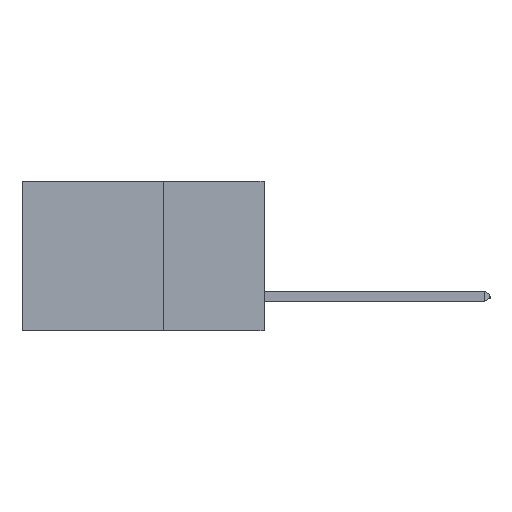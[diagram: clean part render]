
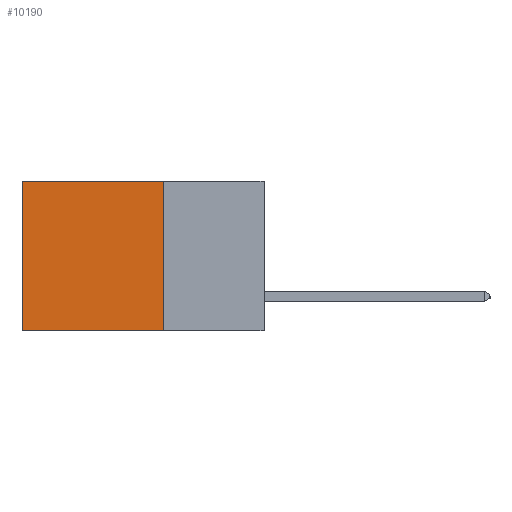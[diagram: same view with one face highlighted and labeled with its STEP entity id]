
A CAD part, left-side view. The second image highlights one B-rep face of the part: STEP entity #10190.
In plain terms, the highlighted planar face has unit normal (-1, 0, 0).
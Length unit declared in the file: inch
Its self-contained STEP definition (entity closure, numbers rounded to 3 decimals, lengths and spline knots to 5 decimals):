
#418 = DIRECTION ( 'NONE',  ( 0., 0., -1. ) ) ;
#2189 = LINE ( 'NONE', #14731, #21818 ) ;
#2745 = VECTOR ( 'NONE', #11582, 39.37008 ) ;
#2777 = VERTEX_POINT ( 'NONE', #9541 ) ;
#3739 = DIRECTION ( 'NONE',  ( 0., 1., 0. ) ) ;
#4799 = CARTESIAN_POINT ( 'NONE',  ( 0.298, 0.25, 0. ) ) ;
#5933 = EDGE_CURVE ( 'NONE', #11827, #14405, #5958, .T. ) ;
#5958 = LINE ( 'NONE', #19879, #7704 ) ;
#7068 = ORIENTED_EDGE ( 'NONE', *, *, #18054, .F. ) ;
#7145 = EDGE_CURVE ( 'NONE', #2777, #14405, #16252, .T. ) ;
#7150 = EDGE_LOOP ( 'NONE', ( #20111, #16093, #7068, #17313 ) ) ;
#7327 = CARTESIAN_POINT ( 'NONE',  ( 0.298, 0.25, 0. ) ) ;
#7704 = VECTOR ( 'NONE', #14851, 39.37008 ) ;
#9541 = CARTESIAN_POINT ( 'NONE',  ( 0.298, 0.25, -0.37 ) ) ;
#10190 = ADVANCED_FACE ( 'NONE', ( #22215 ), #18770, .F. ) ;
#11484 = DIRECTION ( 'NONE',  ( 1., 0., 0. ) ) ;
#11582 = DIRECTION ( 'NONE',  ( 0., 1., 0. ) ) ;
#11827 = VERTEX_POINT ( 'NONE', #17810 ) ;
#13732 = LINE ( 'NONE', #4799, #22998 ) ;
#14405 = VERTEX_POINT ( 'NONE', #16106 ) ;
#14731 = CARTESIAN_POINT ( 'NONE',  ( 0.298, 0.25, 0. ) ) ;
#14851 = DIRECTION ( 'NONE',  ( 0., 0., -1. ) ) ;
#15827 = DIRECTION ( 'NONE',  ( 0., 0., -1. ) ) ;
#16093 = ORIENTED_EDGE ( 'NONE', *, *, #7145, .F. ) ;
#16106 = CARTESIAN_POINT ( 'NONE',  ( 0.298, 0.6, -0.37 ) ) ;
#16252 = LINE ( 'NONE', #22608, #2745 ) ;
#16518 = VERTEX_POINT ( 'NONE', #7327 ) ;
#17313 = ORIENTED_EDGE ( 'NONE', *, *, #18981, .T. ) ;
#17810 = CARTESIAN_POINT ( 'NONE',  ( 0.298, 0.6, 0. ) ) ;
#18054 = EDGE_CURVE ( 'NONE', #16518, #2777, #13732, .T. ) ;
#18770 = PLANE ( 'NONE',  #23644 ) ;
#18981 = EDGE_CURVE ( 'NONE', #16518, #11827, #2189, .T. ) ;
#19879 = CARTESIAN_POINT ( 'NONE',  ( 0.298, 0.6, 0. ) ) ;
#20111 = ORIENTED_EDGE ( 'NONE', *, *, #5933, .T. ) ;
#21818 = VECTOR ( 'NONE', #3739, 39.37008 ) ;
#22215 = FACE_OUTER_BOUND ( 'NONE', #7150, .T. ) ;
#22506 = CARTESIAN_POINT ( 'NONE',  ( 0.298, 0.25, 0. ) ) ;
#22608 = CARTESIAN_POINT ( 'NONE',  ( 0.298, 0.25, -0.37 ) ) ;
#22998 = VECTOR ( 'NONE', #15827, 39.37008 ) ;
#23644 = AXIS2_PLACEMENT_3D ( 'NONE', #22506, #11484, #418 ) ;
